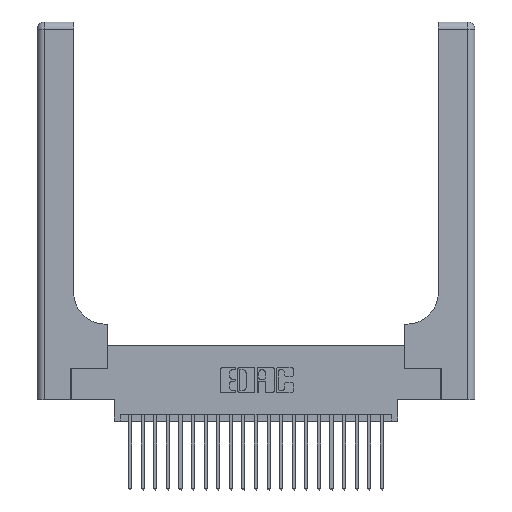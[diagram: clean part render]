
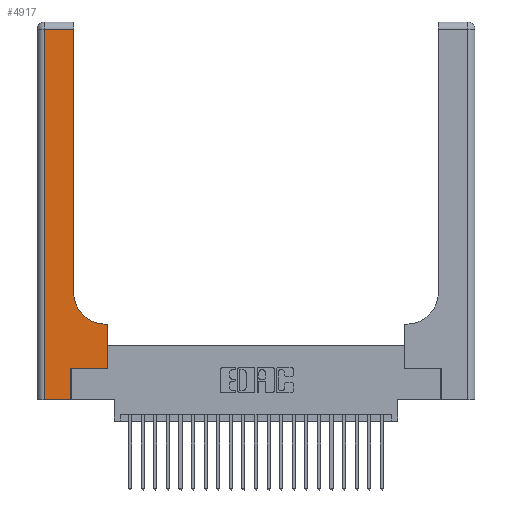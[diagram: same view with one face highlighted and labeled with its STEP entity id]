
A CAD part, top view. The second image highlights one B-rep face of the part: STEP entity #4917.
In plain terms, the highlighted planar face has unit normal (0, 0, 1).
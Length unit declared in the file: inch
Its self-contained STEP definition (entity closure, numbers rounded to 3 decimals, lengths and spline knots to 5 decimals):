
#39 = CARTESIAN_POINT ( 'NONE',  ( 0.5585, 0.25, 0.37 ) ) ;
#263 = DIRECTION ( 'NONE',  ( 1., 0., 0. ) ) ;
#360 = DIRECTION ( 'NONE',  ( -1., 0., 0. ) ) ;
#603 = VECTOR ( 'NONE', #360, 39.37008 ) ;
#939 = CARTESIAN_POINT ( 'NONE',  ( 0.269, 0., 0.37 ) ) ;
#1075 = LINE ( 'NONE', #5893, #20720 ) ;
#2054 = LINE ( 'NONE', #6253, #16353 ) ;
#2107 = LINE ( 'NONE', #6866, #17320 ) ;
#2143 = AXIS2_PLACEMENT_3D ( 'NONE', #13511, #23259, #4055 ) ;
#2192 = CARTESIAN_POINT ( 'NONE',  ( 0.2915, 0.6, 0.37 ) ) ;
#2414 = CARTESIAN_POINT ( 'NONE',  ( 0.06, 0., 0.37 ) ) ;
#3887 = VERTEX_POINT ( 'NONE', #6368 ) ;
#4055 = DIRECTION ( 'NONE',  ( -1., 0., 0. ) ) ;
#4126 = VERTEX_POINT ( 'NONE', #16464 ) ;
#4532 = EDGE_CURVE ( 'NONE', #15935, #24399, #6031, .T. ) ;
#4640 = CARTESIAN_POINT ( 'NONE',  ( 0.269, 0.25, 0.37 ) ) ;
#4917 = ADVANCED_FACE ( 'NONE', ( #22727 ), #13672, .F. ) ;
#5047 = LINE ( 'NONE', #15459, #603 ) ;
#5684 = EDGE_CURVE ( 'NONE', #16108, #4126, #2107, .T. ) ;
#5893 = CARTESIAN_POINT ( 'NONE',  ( 0.06, 3., 0.37 ) ) ;
#6031 = LINE ( 'NONE', #6789, #15588 ) ;
#6253 = CARTESIAN_POINT ( 'NONE',  ( 0., 0., 0.37 ) ) ;
#6368 = CARTESIAN_POINT ( 'NONE',  ( 0.5415, 0.6, 0.37 ) ) ;
#6411 = EDGE_CURVE ( 'NONE', #3887, #16108, #22653, .T. ) ;
#6789 = CARTESIAN_POINT ( 'NONE',  ( 0.269, 0., 0.37 ) ) ;
#6866 = CARTESIAN_POINT ( 'NONE',  ( 0.2915, 3., 0.37 ) ) ;
#6873 = ORIENTED_EDGE ( 'NONE', *, *, #11569, .T. ) ;
#7511 = EDGE_CURVE ( 'NONE', #21445, #11133, #24610, .T. ) ;
#7765 = DIRECTION ( 'NONE',  ( 0., 0., -1. ) ) ;
#8338 = DIRECTION ( 'NONE',  ( 1., 0., 0. ) ) ;
#8397 = DIRECTION ( 'NONE',  ( 0., 1., 0. ) ) ;
#11133 = VERTEX_POINT ( 'NONE', #23478 ) ;
#11569 = EDGE_CURVE ( 'NONE', #24399, #21445, #16699, .T. ) ;
#11634 = VECTOR ( 'NONE', #19752, 39.37008 ) ;
#12035 = ORIENTED_EDGE ( 'NONE', *, *, #19269, .T. ) ;
#13511 = CARTESIAN_POINT ( 'NONE',  ( 0., 3., 0.37 ) ) ;
#13672 = PLANE ( 'NONE',  #2143 ) ;
#13993 = VERTEX_POINT ( 'NONE', #2414 ) ;
#14276 = DIRECTION ( 'NONE',  ( 0., 1., 0. ) ) ;
#14510 = VECTOR ( 'NONE', #17280, 39.37008 ) ;
#14989 = ORIENTED_EDGE ( 'NONE', *, *, #4532, .T. ) ;
#14993 = CARTESIAN_POINT ( 'NONE',  ( 0.269, 0.25, 0.37 ) ) ;
#14995 = ORIENTED_EDGE ( 'NONE', *, *, #15770, .T. ) ;
#15397 = VECTOR ( 'NONE', #8397, 39.37008 ) ;
#15459 = CARTESIAN_POINT ( 'NONE',  ( 0., 2.94, 0.37 ) ) ;
#15588 = VECTOR ( 'NONE', #20575, 39.37008 ) ;
#15770 = EDGE_CURVE ( 'NONE', #13993, #15935, #2054, .T. ) ;
#15790 = VERTEX_POINT ( 'NONE', #23118 ) ;
#15883 = ORIENTED_EDGE ( 'NONE', *, *, #5684, .T. ) ;
#15935 = VERTEX_POINT ( 'NONE', #939 ) ;
#16108 = VERTEX_POINT ( 'NONE', #20576 ) ;
#16353 = VECTOR ( 'NONE', #8338, 39.37008 ) ;
#16464 = CARTESIAN_POINT ( 'NONE',  ( 0.2915, 2.94, 0.37 ) ) ;
#16699 = LINE ( 'NONE', #4640, #11634 ) ;
#17126 = CARTESIAN_POINT ( 'NONE',  ( 0.5415, 0.85, 0.37 ) ) ;
#17198 = EDGE_CURVE ( 'NONE', #11133, #3887, #20464, .T. ) ;
#17207 = ORIENTED_EDGE ( 'NONE', *, *, #6411, .T. ) ;
#17280 = DIRECTION ( 'NONE',  ( -1., 0., 0. ) ) ;
#17320 = VECTOR ( 'NONE', #14276, 39.37008 ) ;
#17914 = EDGE_CURVE ( 'NONE', #15790, #13993, #1075, .T. ) ;
#18036 = ORIENTED_EDGE ( 'NONE', *, *, #17914, .T. ) ;
#18237 = CARTESIAN_POINT ( 'NONE',  ( 0.5585, 0.25, 0.37 ) ) ;
#19172 = AXIS2_PLACEMENT_3D ( 'NONE', #17126, #7765, #263 ) ;
#19269 = EDGE_CURVE ( 'NONE', #4126, #15790, #5047, .T. ) ;
#19752 = DIRECTION ( 'NONE',  ( 1., 0., 0. ) ) ;
#20464 = LINE ( 'NONE', #2192, #14510 ) ;
#20575 = DIRECTION ( 'NONE',  ( 0., 1., 0. ) ) ;
#20576 = CARTESIAN_POINT ( 'NONE',  ( 0.2915, 0.85, 0.37 ) ) ;
#20720 = VECTOR ( 'NONE', #21225, 39.37008 ) ;
#21225 = DIRECTION ( 'NONE',  ( 0., -1., 0. ) ) ;
#21445 = VERTEX_POINT ( 'NONE', #39 ) ;
#22653 = CIRCLE ( 'NONE', #19172, 0.25 ) ;
#22727 = FACE_OUTER_BOUND ( 'NONE', #23375, .T. ) ;
#23118 = CARTESIAN_POINT ( 'NONE',  ( 0.06, 2.94, 0.37 ) ) ;
#23194 = ORIENTED_EDGE ( 'NONE', *, *, #17198, .T. ) ;
#23259 = DIRECTION ( 'NONE',  ( 0., 0., -1. ) ) ;
#23375 = EDGE_LOOP ( 'NONE', ( #15883, #12035, #18036, #14995, #14989, #6873, #24286, #23194, #17207 ) ) ;
#23478 = CARTESIAN_POINT ( 'NONE',  ( 0.5585, 0.6, 0.37 ) ) ;
#24286 = ORIENTED_EDGE ( 'NONE', *, *, #7511, .T. ) ;
#24399 = VERTEX_POINT ( 'NONE', #14993 ) ;
#24610 = LINE ( 'NONE', #18237, #15397 ) ;
